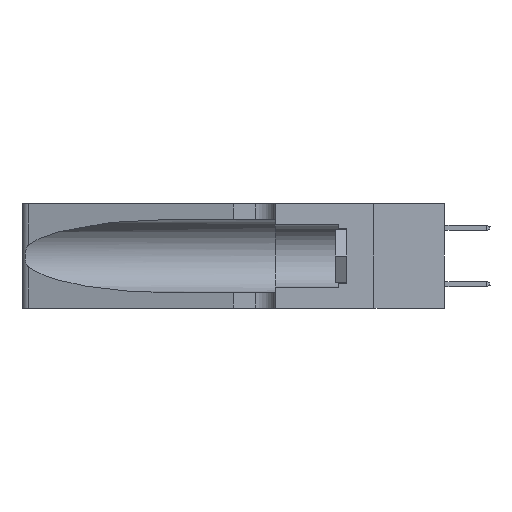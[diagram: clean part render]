
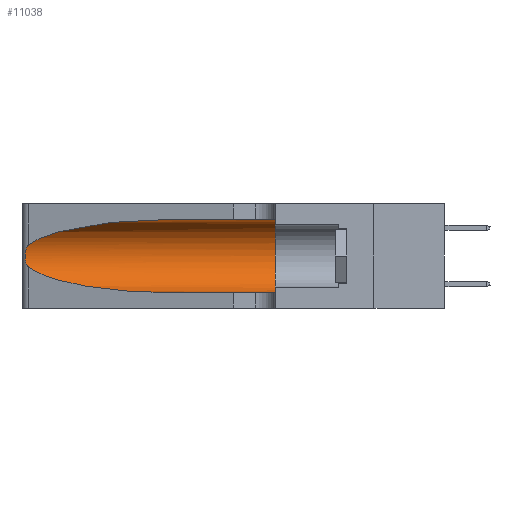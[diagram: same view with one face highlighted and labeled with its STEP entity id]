
A CAD part, left-side view. The second image highlights one B-rep face of the part: STEP entity #11038.
In plain terms, the highlighted cylindrical face has radius 3.308 mm (diameter 6.617 mm), a partial arc.
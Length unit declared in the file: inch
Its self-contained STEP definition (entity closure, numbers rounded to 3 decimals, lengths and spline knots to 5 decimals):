
#120 = DIRECTION ( 'NONE',  ( 0., 1., 0. ) ) ;
#766 = DIRECTION ( 'NONE',  ( 0., -1., 0. ) ) ;
#1193 = CARTESIAN_POINT ( 'NONE',  ( 0.1305, 0.72297, 0.31525 ) ) ;
#1194 = VECTOR ( 'NONE', #766, 39.37008 ) ;
#2066 = CARTESIAN_POINT ( 'NONE',  ( 0.18966, 0.96281, 0.05475 ) ) ;
#2163 = CARTESIAN_POINT ( 'NONE',  ( 0.1305, 1.61858, 0.05475 ) ) ;
#2272 = CARTESIAN_POINT ( 'NONE',  ( 0.25487, 1.22718, 0.14631 ) ) ;
#2358 = CYLINDRICAL_SURFACE ( 'NONE', #20260, 0.13025 ) ;
#3183 = EDGE_CURVE ( 'NONE', #10970, #5889, #18182, .T. ) ;
#3255 = EDGE_CURVE ( 'NONE', #10970, #21713, #8313, .T. ) ;
#5259 = ORIENTED_EDGE ( 'NONE', *, *, #3255, .F. ) ;
#5333 = DIRECTION ( 'NONE',  ( 0., 0., -1. ) ) ;
#5456 = EDGE_CURVE ( 'NONE', #21713, #24576, #27113, .T. ) ;
#5528 = CARTESIAN_POINT ( 'NONE',  ( 0.25854, 1.2359, 0.20912 ) ) ;
#5634 = CARTESIAN_POINT ( 'NONE',  ( 0.26075, 1.23896, 0.19203 ) ) ;
#5889 = VERTEX_POINT ( 'NONE', #16725 ) ;
#5905 = EDGE_LOOP ( 'NONE', ( #9148, #22702, #13761, #22283, #21960, #5259 ) ) ;
#6544 = CARTESIAN_POINT ( 'NONE',  ( 0.25487, 1.22718, 0.14631 ) ) ;
#7240 = CARTESIAN_POINT ( 'NONE',  ( 0.25487, 1.22718, 0.22369 ) ) ;
#7697 = LINE ( 'NONE', #2163, #11603 ) ;
#7819 = CARTESIAN_POINT ( 'NONE',  ( 0.26018, 1.23835, 0.19895 ) ) ;
#8313 = LINE ( 'NONE', #13676, #1194 ) ;
#8331 = CARTESIAN_POINT ( 'NONE',  ( 0.18966, 0.96281, 0.31525 ) ) ;
#8725 = FACE_OUTER_BOUND ( 'NONE', #5905, .T. ) ;
#9112 = EDGE_CURVE ( 'NONE', #25515, #28958, #28773, .T. ) ;
#9148 = ORIENTED_EDGE ( 'NONE', *, *, #3183, .T. ) ;
#10487 = CARTESIAN_POINT ( 'NONE',  ( 0.25639, 1.23186, 0.15144 ) ) ;
#10970 = VERTEX_POINT ( 'NONE', #12699 ) ;
#11038 = ADVANCED_FACE ( 'NONE', ( #8725 ), #2358, .F. ) ;
#11603 = VECTOR ( 'NONE', #24844, 39.37008 ) ;
#12699 = CARTESIAN_POINT ( 'NONE',  ( 0.1305, 0.72297, 0.31525 ) ) ;
#13047 = CARTESIAN_POINT ( 'NONE',  ( 0.1305, 0.35, 0.31525 ) ) ;
#13144 = EDGE_CURVE ( 'NONE', #28958, #24576, #7697, .T. ) ;
#13287 = CARTESIAN_POINT ( 'NONE',  ( 0.1305, 1.61858, 0.185 ) ) ;
#13541 = EDGE_CURVE ( 'NONE', #5889, #25515, #14742, .T. ) ;
#13676 = CARTESIAN_POINT ( 'NONE',  ( 0.1305, 1.61858, 0.31525 ) ) ;
#13761 = ORIENTED_EDGE ( 'NONE', *, *, #9112, .T. ) ;
#14742 = B_SPLINE_CURVE_WITH_KNOTS ( 'NONE', 3,
 ( #7240, #21284, #19420, #25843, #5528, #7819, #5634, #19911, #21990, #15253, #24062, #10487, #15043, #17728 ),
 .UNSPECIFIED., .F., .F.,
 ( 4, 2, 2, 2, 2, 2, 4 ),
 ( 0., 0.00027, 0.00053, 0.00107, 0.0016, 0.00187, 0.00214 ),
 .UNSPECIFIED. ) ;
#15043 = CARTESIAN_POINT ( 'NONE',  ( 0.25555, 1.22993, 0.14849 ) ) ;
#15212 = CARTESIAN_POINT ( 'NONE',  ( 0.1305, 0.35, 0.05475 ) ) ;
#15253 = CARTESIAN_POINT ( 'NONE',  ( 0.25856, 1.23593, 0.16098 ) ) ;
#16110 = DIRECTION ( 'NONE',  ( 0., 0., 1. ) ) ;
#16725 = CARTESIAN_POINT ( 'NONE',  ( 0.25487, 1.22718, 0.22369 ) ) ;
#17080 = CARTESIAN_POINT ( 'NONE',  ( 0.25487, 1.22718, 0.22369 ) ) ;
#17728 = CARTESIAN_POINT ( 'NONE',  ( 0.25487, 1.22718, 0.14631 ) ) ;
#17847 = CARTESIAN_POINT ( 'NONE',  ( 0.1305, 0.72297, 0.05475 ) ) ;
#17948 = CARTESIAN_POINT ( 'NONE',  ( 0.2373, 1.15595, 0.08982 ) ) ;
#18182 =( BOUNDED_CURVE ( )  B_SPLINE_CURVE ( 3, ( #1193, #8331, #21601, #17080 ),
 .UNSPECIFIED., .F., .F. ) 
 B_SPLINE_CURVE_WITH_KNOTS ( ( 4, 4 ),
 ( 1.5708, 2.84003 ),
 .UNSPECIFIED. ) 
 CURVE ( )  GEOMETRIC_REPRESENTATION_ITEM ( )  RATIONAL_B_SPLINE_CURVE ( ( 1., 0.87, 0.87, 1. ) ) 
 REPRESENTATION_ITEM ( '' )  );
#18800 = AXIS2_PLACEMENT_3D ( 'NONE', #27284, #120, #16110 ) ;
#19167 = CARTESIAN_POINT ( 'NONE',  ( 0.1305, 0.72297, 0.05475 ) ) ;
#19420 = CARTESIAN_POINT ( 'NONE',  ( 0.25639, 1.23184, 0.21858 ) ) ;
#19911 = CARTESIAN_POINT ( 'NONE',  ( 0.26075, 1.23896, 0.178 ) ) ;
#20260 = AXIS2_PLACEMENT_3D ( 'NONE', #13287, #22954, #5333 ) ;
#21284 = CARTESIAN_POINT ( 'NONE',  ( 0.25555, 1.22994, 0.2215 ) ) ;
#21601 = CARTESIAN_POINT ( 'NONE',  ( 0.2373, 1.15595, 0.28018 ) ) ;
#21713 = VERTEX_POINT ( 'NONE', #13047 ) ;
#21960 = ORIENTED_EDGE ( 'NONE', *, *, #5456, .F. ) ;
#21990 = CARTESIAN_POINT ( 'NONE',  ( 0.26017, 1.23833, 0.17102 ) ) ;
#22283 = ORIENTED_EDGE ( 'NONE', *, *, #13144, .T. ) ;
#22702 = ORIENTED_EDGE ( 'NONE', *, *, #13541, .T. ) ;
#22954 = DIRECTION ( 'NONE',  ( 0., -1., 0. ) ) ;
#24062 = CARTESIAN_POINT ( 'NONE',  ( 0.25789, 1.23486, 0.15765 ) ) ;
#24576 = VERTEX_POINT ( 'NONE', #15212 ) ;
#24844 = DIRECTION ( 'NONE',  ( 0., -1., 0. ) ) ;
#25515 = VERTEX_POINT ( 'NONE', #2272 ) ;
#25843 = CARTESIAN_POINT ( 'NONE',  ( 0.25787, 1.23484, 0.2124 ) ) ;
#27113 = CIRCLE ( 'NONE', #18800, 0.13025 ) ;
#27284 = CARTESIAN_POINT ( 'NONE',  ( 0.1305, 0.35, 0.185 ) ) ;
#28773 =( BOUNDED_CURVE ( )  B_SPLINE_CURVE ( 3, ( #6544, #17948, #2066, #17847 ),
 .UNSPECIFIED., .F., .F. ) 
 B_SPLINE_CURVE_WITH_KNOTS ( ( 4, 4 ),
 ( 3.44316, 4.71239 ),
 .UNSPECIFIED. ) 
 CURVE ( )  GEOMETRIC_REPRESENTATION_ITEM ( )  RATIONAL_B_SPLINE_CURVE ( ( 1., 0.87, 0.87, 1. ) ) 
 REPRESENTATION_ITEM ( '' )  );
#28958 = VERTEX_POINT ( 'NONE', #19167 ) ;
